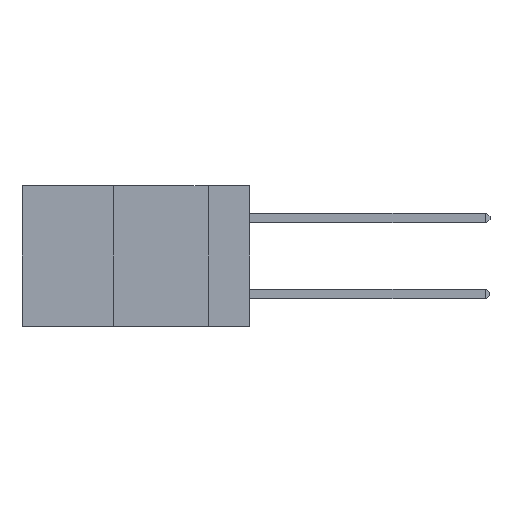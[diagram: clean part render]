
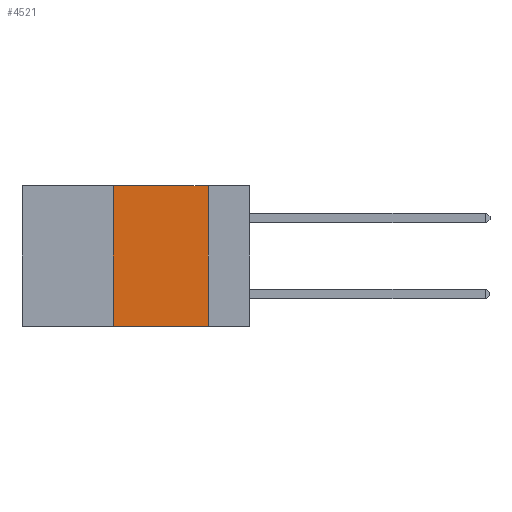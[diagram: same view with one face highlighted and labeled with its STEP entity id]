
A CAD part, left-side view. The second image highlights one B-rep face of the part: STEP entity #4521.
In plain terms, the highlighted planar face has unit normal (-1, 0, 0).
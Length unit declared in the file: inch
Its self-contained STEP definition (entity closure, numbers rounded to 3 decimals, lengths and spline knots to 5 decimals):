
#1764 = AXIS2_PLACEMENT_3D ( 'NONE', #16823, #15337, #6118 ) ;
#2704 = EDGE_CURVE ( 'NONE', #18069, #18382, #6982, .T. ) ;
#2762 = DIRECTION ( 'NONE',  ( 0., 0., 1. ) ) ;
#3050 = DIRECTION ( 'NONE',  ( 0., 0., -1. ) ) ;
#3271 = CARTESIAN_POINT ( 'NONE',  ( 0., 0.6, 0. ) ) ;
#3574 = DIRECTION ( 'NONE',  ( 0., -1., 0. ) ) ;
#3802 = EDGE_CURVE ( 'NONE', #18069, #15609, #5012, .T. ) ;
#3957 = CARTESIAN_POINT ( 'NONE',  ( 0., 0.6, -0.37 ) ) ;
#4447 = CARTESIAN_POINT ( 'NONE',  ( 0., 0.36, -0.37 ) ) ;
#4521 = ADVANCED_FACE ( 'NONE', ( #15214 ), #13785, .F. ) ;
#4778 = DIRECTION ( 'NONE',  ( 0., -1., 0. ) ) ;
#5012 = LINE ( 'NONE', #10608, #16817 ) ;
#5782 = CARTESIAN_POINT ( 'NONE',  ( 0., 0.11, 0. ) ) ;
#5954 = EDGE_CURVE ( 'NONE', #19783, #18382, #10119, .T. ) ;
#6118 = DIRECTION ( 'NONE',  ( 0., 0., -1. ) ) ;
#6982 = LINE ( 'NONE', #3957, #10616 ) ;
#9635 = VECTOR ( 'NONE', #3050, 39.37008 ) ;
#9939 = CARTESIAN_POINT ( 'NONE',  ( 0., 0.11, -0.37 ) ) ;
#10119 = LINE ( 'NONE', #20011, #9635 ) ;
#10608 = CARTESIAN_POINT ( 'NONE',  ( 0., 0.36, 0. ) ) ;
#10616 = VECTOR ( 'NONE', #3574, 39.37008 ) ;
#10810 = ORIENTED_EDGE ( 'NONE', *, *, #3802, .F. ) ;
#10938 = CARTESIAN_POINT ( 'NONE',  ( 0., 0.36, 0. ) ) ;
#12751 = ORIENTED_EDGE ( 'NONE', *, *, #18888, .F. ) ;
#13785 = PLANE ( 'NONE',  #1764 ) ;
#15214 = FACE_OUTER_BOUND ( 'NONE', #18421, .T. ) ;
#15337 = DIRECTION ( 'NONE',  ( 1., 0., 0. ) ) ;
#15609 = VERTEX_POINT ( 'NONE', #10938 ) ;
#16817 = VECTOR ( 'NONE', #2762, 39.37008 ) ;
#16823 = CARTESIAN_POINT ( 'NONE',  ( 0., 0.6, 0. ) ) ;
#17997 = ORIENTED_EDGE ( 'NONE', *, *, #2704, .T. ) ;
#18002 = ORIENTED_EDGE ( 'NONE', *, *, #5954, .F. ) ;
#18069 = VERTEX_POINT ( 'NONE', #4447 ) ;
#18382 = VERTEX_POINT ( 'NONE', #9939 ) ;
#18421 = EDGE_LOOP ( 'NONE', ( #18002, #12751, #10810, #17997 ) ) ;
#18427 = VECTOR ( 'NONE', #4778, 39.37008 ) ;
#18888 = EDGE_CURVE ( 'NONE', #15609, #19783, #18931, .T. ) ;
#18931 = LINE ( 'NONE', #3271, #18427 ) ;
#19783 = VERTEX_POINT ( 'NONE', #5782 ) ;
#20011 = CARTESIAN_POINT ( 'NONE',  ( 0., 0.11, 0. ) ) ;
